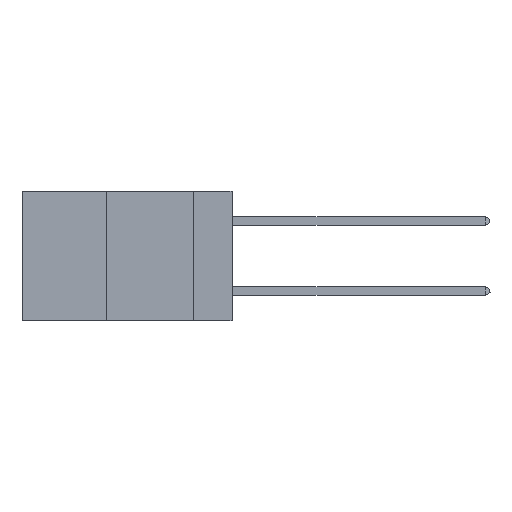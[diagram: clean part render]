
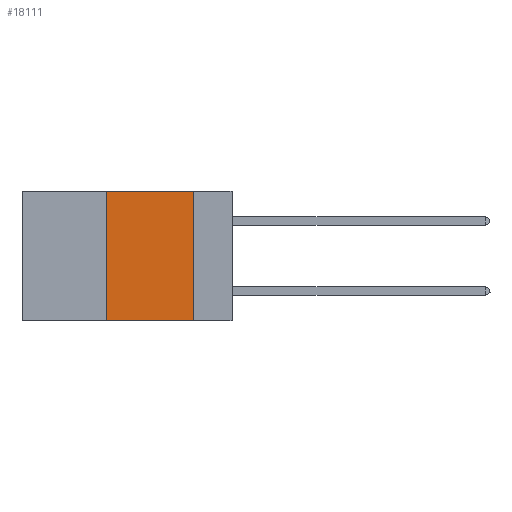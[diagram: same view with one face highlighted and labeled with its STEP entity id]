
A CAD part, left-side view. The second image highlights one B-rep face of the part: STEP entity #18111.
In plain terms, the highlighted planar face has unit normal (-1, 0, 0).
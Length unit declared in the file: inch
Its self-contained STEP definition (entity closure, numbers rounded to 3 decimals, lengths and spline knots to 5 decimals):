
#388 = ORIENTED_EDGE ( 'NONE', *, *, #7244, .F. ) ;
#3953 = CARTESIAN_POINT ( 'NONE',  ( 0., 0.36, 0. ) ) ;
#5584 = CARTESIAN_POINT ( 'NONE',  ( 0., 0.11, 0. ) ) ;
#6390 = VECTOR ( 'NONE', #23482, 39.37008 ) ;
#7244 = EDGE_CURVE ( 'NONE', #10588, #24483, #29862, .T. ) ;
#7411 = ORIENTED_EDGE ( 'NONE', *, *, #19219, .F. ) ;
#7710 = PLANE ( 'NONE',  #34494 ) ;
#8302 = DIRECTION ( 'NONE',  ( 0., -1., 0. ) ) ;
#8358 = EDGE_CURVE ( 'NONE', #22422, #10588, #39967, .T. ) ;
#8431 = CARTESIAN_POINT ( 'NONE',  ( 0., 0.6, -0.37 ) ) ;
#9008 = CARTESIAN_POINT ( 'NONE',  ( 0., 0.11, -0.37 ) ) ;
#9156 = DIRECTION ( 'NONE',  ( 0., 0., -1. ) ) ;
#10178 = LINE ( 'NONE', #8431, #28102 ) ;
#10588 = VERTEX_POINT ( 'NONE', #15451 ) ;
#13942 = LINE ( 'NONE', #3953, #36793 ) ;
#14326 = FACE_OUTER_BOUND ( 'NONE', #29383, .T. ) ;
#15323 = ORIENTED_EDGE ( 'NONE', *, *, #37079, .T. ) ;
#15451 = CARTESIAN_POINT ( 'NONE',  ( 0., 0.11, 0. ) ) ;
#15771 = VECTOR ( 'NONE', #9156, 39.37008 ) ;
#18111 = ADVANCED_FACE ( 'NONE', ( #14326 ), #7710, .F. ) ;
#19219 = EDGE_CURVE ( 'NONE', #20891, #22422, #13942, .T. ) ;
#20521 = CARTESIAN_POINT ( 'NONE',  ( 0., 0.6, 0. ) ) ;
#20891 = VERTEX_POINT ( 'NONE', #22818 ) ;
#22422 = VERTEX_POINT ( 'NONE', #37239 ) ;
#22818 = CARTESIAN_POINT ( 'NONE',  ( 0., 0.36, -0.37 ) ) ;
#23482 = DIRECTION ( 'NONE',  ( 0., -1., 0. ) ) ;
#23584 = ORIENTED_EDGE ( 'NONE', *, *, #8358, .F. ) ;
#24483 = VERTEX_POINT ( 'NONE', #9008 ) ;
#26734 = CARTESIAN_POINT ( 'NONE',  ( 0., 0.6, 0. ) ) ;
#28102 = VECTOR ( 'NONE', #8302, 39.37008 ) ;
#29383 = EDGE_LOOP ( 'NONE', ( #388, #23584, #7411, #15323 ) ) ;
#29464 = DIRECTION ( 'NONE',  ( 1., 0., 0. ) ) ;
#29613 = DIRECTION ( 'NONE',  ( 0., 0., -1. ) ) ;
#29862 = LINE ( 'NONE', #5584, #15771 ) ;
#32134 = DIRECTION ( 'NONE',  ( 0., 0., 1. ) ) ;
#34494 = AXIS2_PLACEMENT_3D ( 'NONE', #20521, #29464, #29613 ) ;
#36793 = VECTOR ( 'NONE', #32134, 39.37008 ) ;
#37079 = EDGE_CURVE ( 'NONE', #20891, #24483, #10178, .T. ) ;
#37239 = CARTESIAN_POINT ( 'NONE',  ( 0., 0.36, 0. ) ) ;
#39967 = LINE ( 'NONE', #26734, #6390 ) ;
